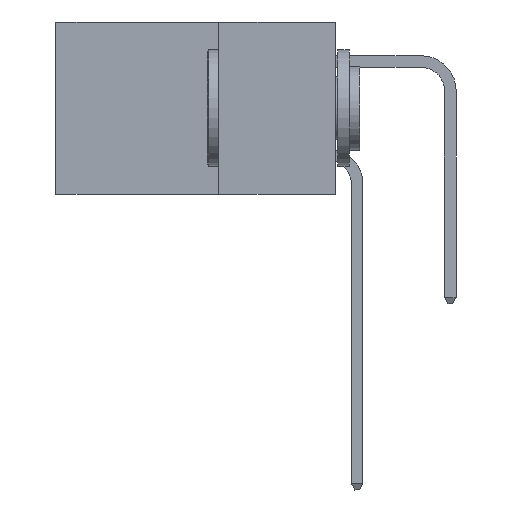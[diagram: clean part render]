
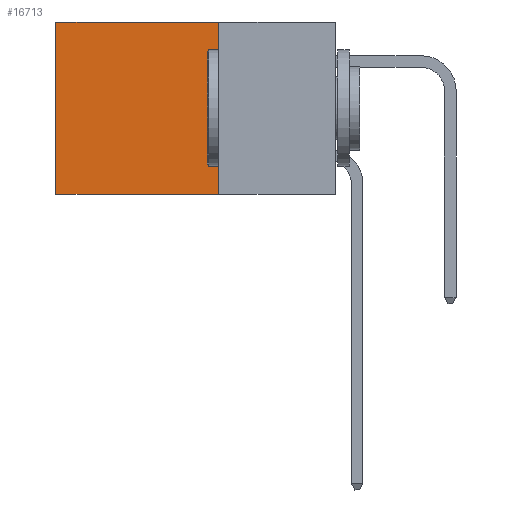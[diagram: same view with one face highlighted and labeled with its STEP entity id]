
A CAD part, left-side view. The second image highlights one B-rep face of the part: STEP entity #16713.
In plain terms, the highlighted planar face has unit normal (-1, 0, 0).
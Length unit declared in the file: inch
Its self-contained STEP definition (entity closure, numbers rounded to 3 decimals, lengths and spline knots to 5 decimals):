
#42 = EDGE_CURVE ( 'NONE', #24785, #36836, #10925, .T. ) ;
#2492 = VECTOR ( 'NONE', #10007, 39.37008 ) ;
#2689 = CARTESIAN_POINT ( 'NONE',  ( 0.2875, 0.6, -0.37 ) ) ;
#3945 = DIRECTION ( 'NONE',  ( 0., 0., -1. ) ) ;
#4889 = EDGE_CURVE ( 'NONE', #36905, #36836, #36400, .T. ) ;
#7510 = AXIS2_PLACEMENT_3D ( 'NONE', #10173, #22721, #3945 ) ;
#8009 = CARTESIAN_POINT ( 'NONE',  ( 0.2875, 0.25, -0.37 ) ) ;
#8625 = CARTESIAN_POINT ( 'NONE',  ( 0.2875, 0.25, 0. ) ) ;
#9462 = CARTESIAN_POINT ( 'NONE',  ( 0.2875, 0.6, 0. ) ) ;
#10007 = DIRECTION ( 'NONE',  ( 0., 1., 0. ) ) ;
#10173 = CARTESIAN_POINT ( 'NONE',  ( 0.2875, 0.25, 0. ) ) ;
#10925 = LINE ( 'NONE', #31829, #2492 ) ;
#11092 = FACE_OUTER_BOUND ( 'NONE', #39866, .T. ) ;
#12852 = LINE ( 'NONE', #24319, #28504 ) ;
#13534 = ORIENTED_EDGE ( 'NONE', *, *, #25393, .T. ) ;
#14840 = LINE ( 'NONE', #20241, #21175 ) ;
#16104 = ORIENTED_EDGE ( 'NONE', *, *, #35510, .F. ) ;
#16713 = ADVANCED_FACE ( 'NONE', ( #11092 ), #31998, .F. ) ;
#17709 = CARTESIAN_POINT ( 'NONE',  ( 0.2875, 0.6, 0. ) ) ;
#18421 = VERTEX_POINT ( 'NONE', #8625 ) ;
#20241 = CARTESIAN_POINT ( 'NONE',  ( 0.2875, 0.25, 0. ) ) ;
#20849 = DIRECTION ( 'NONE',  ( 0., 0., -1. ) ) ;
#21175 = VECTOR ( 'NONE', #23251, 39.37008 ) ;
#22721 = DIRECTION ( 'NONE',  ( 1., 0., 0. ) ) ;
#23251 = DIRECTION ( 'NONE',  ( 0., 1., 0. ) ) ;
#24319 = CARTESIAN_POINT ( 'NONE',  ( 0.2875, 0.25, 0. ) ) ;
#24785 = VERTEX_POINT ( 'NONE', #8009 ) ;
#25393 = EDGE_CURVE ( 'NONE', #18421, #36905, #14840, .T. ) ;
#25559 = ORIENTED_EDGE ( 'NONE', *, *, #4889, .T. ) ;
#26231 = ORIENTED_EDGE ( 'NONE', *, *, #42, .F. ) ;
#27192 = VECTOR ( 'NONE', #20849, 39.37008 ) ;
#27457 = DIRECTION ( 'NONE',  ( 0., 0., -1. ) ) ;
#28504 = VECTOR ( 'NONE', #27457, 39.37008 ) ;
#31829 = CARTESIAN_POINT ( 'NONE',  ( 0.2875, 0.25, -0.37 ) ) ;
#31998 = PLANE ( 'NONE',  #7510 ) ;
#35510 = EDGE_CURVE ( 'NONE', #18421, #24785, #12852, .T. ) ;
#36400 = LINE ( 'NONE', #17709, #27192 ) ;
#36836 = VERTEX_POINT ( 'NONE', #2689 ) ;
#36905 = VERTEX_POINT ( 'NONE', #9462 ) ;
#39866 = EDGE_LOOP ( 'NONE', ( #25559, #26231, #16104, #13534 ) ) ;
